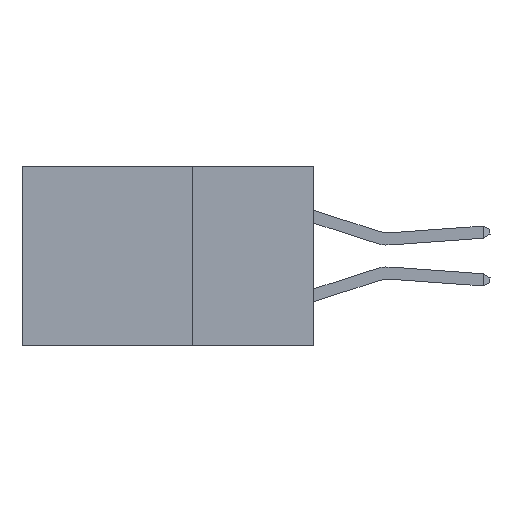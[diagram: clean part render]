
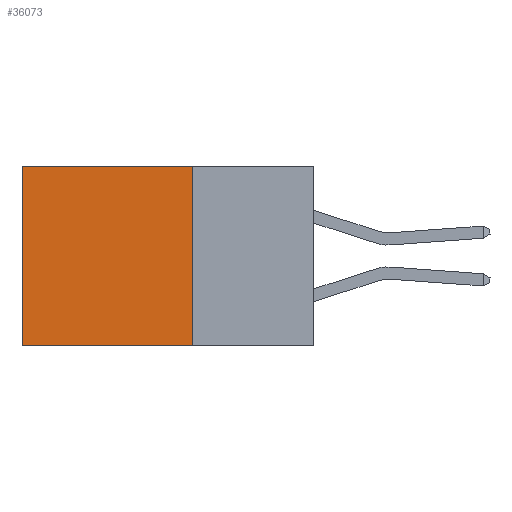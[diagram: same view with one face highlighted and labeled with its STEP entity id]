
A CAD part, left-side view. The second image highlights one B-rep face of the part: STEP entity #36073.
In plain terms, the highlighted planar face has unit normal (-1, 0, 0).
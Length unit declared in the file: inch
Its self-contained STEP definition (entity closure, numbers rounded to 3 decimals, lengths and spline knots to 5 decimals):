
#1211 = VECTOR ( 'NONE', #9739, 39.37008 ) ;
#2262 = EDGE_CURVE ( 'NONE', #32214, #14704, #8742, .T. ) ;
#2360 = LINE ( 'NONE', #27228, #1211 ) ;
#2594 = CARTESIAN_POINT ( 'NONE',  ( 0.2875, 0.6, 0. ) ) ;
#4179 = CARTESIAN_POINT ( 'NONE',  ( 0.2875, 0.25, -0.37 ) ) ;
#5613 = ORIENTED_EDGE ( 'NONE', *, *, #17488, .T. ) ;
#8098 = LINE ( 'NONE', #30165, #25721 ) ;
#8742 = LINE ( 'NONE', #26373, #44718 ) ;
#8756 = ORIENTED_EDGE ( 'NONE', *, *, #14967, .F. ) ;
#9739 = DIRECTION ( 'NONE',  ( 0., 1., 0. ) ) ;
#14704 = VERTEX_POINT ( 'NONE', #4179 ) ;
#14967 = EDGE_CURVE ( 'NONE', #14704, #21621, #8098, .T. ) ;
#17488 = EDGE_CURVE ( 'NONE', #41007, #21621, #34160, .T. ) ;
#19846 = EDGE_LOOP ( 'NONE', ( #5613, #8756, #40557, #28410 ) ) ;
#20366 = FACE_OUTER_BOUND ( 'NONE', #19846, .T. ) ;
#20682 = DIRECTION ( 'NONE',  ( 0., 0., -1. ) ) ;
#21621 = VERTEX_POINT ( 'NONE', #25399 ) ;
#25399 = CARTESIAN_POINT ( 'NONE',  ( 0.2875, 0.6, -0.37 ) ) ;
#25721 = VECTOR ( 'NONE', #40400, 39.37008 ) ;
#26373 = CARTESIAN_POINT ( 'NONE',  ( 0.2875, 0.25, 0. ) ) ;
#27228 = CARTESIAN_POINT ( 'NONE',  ( 0.2875, 0.25, 0. ) ) ;
#28410 = ORIENTED_EDGE ( 'NONE', *, *, #29097, .T. ) ;
#29097 = EDGE_CURVE ( 'NONE', #32214, #41007, #2360, .T. ) ;
#30165 = CARTESIAN_POINT ( 'NONE',  ( 0.2875, 0.25, -0.37 ) ) ;
#31304 = CARTESIAN_POINT ( 'NONE',  ( 0.2875, 0.25, 0. ) ) ;
#32214 = VERTEX_POINT ( 'NONE', #31304 ) ;
#34160 = LINE ( 'NONE', #43222, #35220 ) ;
#34470 = PLANE ( 'NONE',  #39072 ) ;
#34568 = DIRECTION ( 'NONE',  ( 0., 0., -1. ) ) ;
#35220 = VECTOR ( 'NONE', #34568, 39.37008 ) ;
#36073 = ADVANCED_FACE ( 'NONE', ( #20366 ), #34470, .F. ) ;
#37921 = CARTESIAN_POINT ( 'NONE',  ( 0.2875, 0.25, 0. ) ) ;
#39072 = AXIS2_PLACEMENT_3D ( 'NONE', #37921, #41391, #20682 ) ;
#40400 = DIRECTION ( 'NONE',  ( 0., 1., 0. ) ) ;
#40557 = ORIENTED_EDGE ( 'NONE', *, *, #2262, .F. ) ;
#41007 = VERTEX_POINT ( 'NONE', #2594 ) ;
#41391 = DIRECTION ( 'NONE',  ( 1., 0., 0. ) ) ;
#43222 = CARTESIAN_POINT ( 'NONE',  ( 0.2875, 0.6, 0. ) ) ;
#43574 = DIRECTION ( 'NONE',  ( 0., 0., -1. ) ) ;
#44718 = VECTOR ( 'NONE', #43574, 39.37008 ) ;
